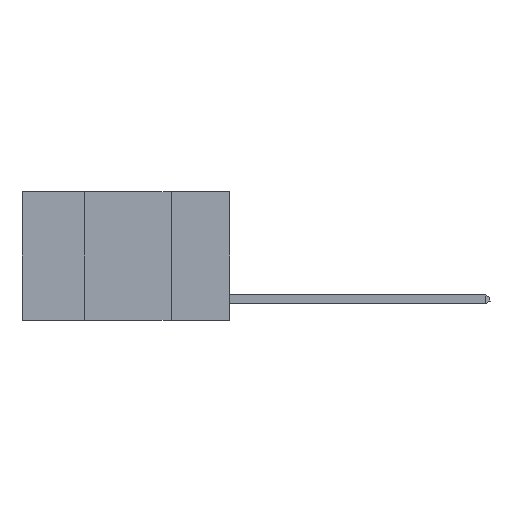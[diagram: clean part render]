
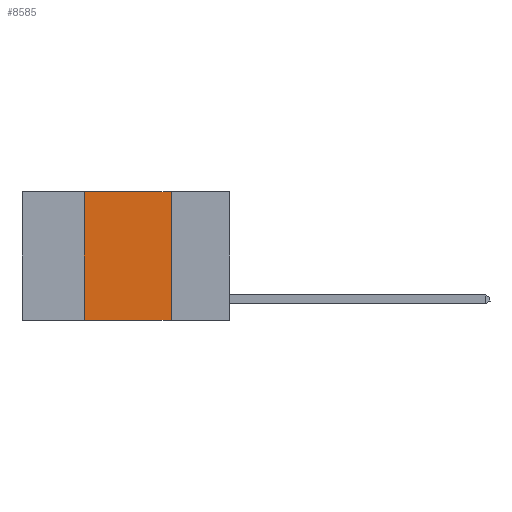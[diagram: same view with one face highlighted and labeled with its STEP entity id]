
A CAD part, left-side view. The second image highlights one B-rep face of the part: STEP entity #8585.
In plain terms, the highlighted planar face has unit normal (-1, 0, 0).
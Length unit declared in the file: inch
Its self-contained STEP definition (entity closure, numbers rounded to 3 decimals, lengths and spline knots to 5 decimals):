
#771 = EDGE_CURVE ( 'NONE', #8509, #4231, #7407, .T. ) ;
#1761 = VERTEX_POINT ( 'NONE', #6417 ) ;
#1877 = AXIS2_PLACEMENT_3D ( 'NONE', #5045, #7422, #2666 ) ;
#2121 = ORIENTED_EDGE ( 'NONE', *, *, #771, .F. ) ;
#2666 = DIRECTION ( 'NONE',  ( 0., 0., -1. ) ) ;
#2999 = EDGE_CURVE ( 'NONE', #1761, #8509, #3537, .T. ) ;
#3537 = LINE ( 'NONE', #6506, #9549 ) ;
#3986 = ORIENTED_EDGE ( 'NONE', *, *, #8775, .F. ) ;
#4179 = CARTESIAN_POINT ( 'NONE',  ( 0., 0.42, 0. ) ) ;
#4231 = VERTEX_POINT ( 'NONE', #6980 ) ;
#4521 = DIRECTION ( 'NONE',  ( 0., -1., 0. ) ) ;
#4941 = FACE_OUTER_BOUND ( 'NONE', #9013, .T. ) ;
#5007 = CARTESIAN_POINT ( 'NONE',  ( 0., 0.17, -0.37 ) ) ;
#5045 = CARTESIAN_POINT ( 'NONE',  ( 0., 0.6, 0. ) ) ;
#5327 = VECTOR ( 'NONE', #8437, 39.37008 ) ;
#5328 = LINE ( 'NONE', #9134, #7410 ) ;
#6099 = CARTESIAN_POINT ( 'NONE',  ( 0., 0.6, -0.37 ) ) ;
#6152 = LINE ( 'NONE', #6099, #7164 ) ;
#6358 = ORIENTED_EDGE ( 'NONE', *, *, #2999, .F. ) ;
#6417 = CARTESIAN_POINT ( 'NONE',  ( 0., 0.42, -0.37 ) ) ;
#6463 = DIRECTION ( 'NONE',  ( 0., 0., 1. ) ) ;
#6506 = CARTESIAN_POINT ( 'NONE',  ( 0., 0.42, 0. ) ) ;
#6622 = PLANE ( 'NONE',  #1877 ) ;
#6980 = CARTESIAN_POINT ( 'NONE',  ( 0., 0.17, 0. ) ) ;
#7164 = VECTOR ( 'NONE', #4521, 39.37008 ) ;
#7407 = LINE ( 'NONE', #9616, #5327 ) ;
#7410 = VECTOR ( 'NONE', #7653, 39.37008 ) ;
#7422 = DIRECTION ( 'NONE',  ( 1., 0., 0. ) ) ;
#7653 = DIRECTION ( 'NONE',  ( 0., 0., -1. ) ) ;
#8396 = ORIENTED_EDGE ( 'NONE', *, *, #8801, .T. ) ;
#8437 = DIRECTION ( 'NONE',  ( 0., -1., 0. ) ) ;
#8509 = VERTEX_POINT ( 'NONE', #4179 ) ;
#8576 = VERTEX_POINT ( 'NONE', #5007 ) ;
#8585 = ADVANCED_FACE ( 'NONE', ( #4941 ), #6622, .F. ) ;
#8775 = EDGE_CURVE ( 'NONE', #4231, #8576, #5328, .T. ) ;
#8801 = EDGE_CURVE ( 'NONE', #1761, #8576, #6152, .T. ) ;
#9013 = EDGE_LOOP ( 'NONE', ( #3986, #2121, #6358, #8396 ) ) ;
#9134 = CARTESIAN_POINT ( 'NONE',  ( 0., 0.17, 0. ) ) ;
#9549 = VECTOR ( 'NONE', #6463, 39.37008 ) ;
#9616 = CARTESIAN_POINT ( 'NONE',  ( 0., 0.6, 0. ) ) ;
